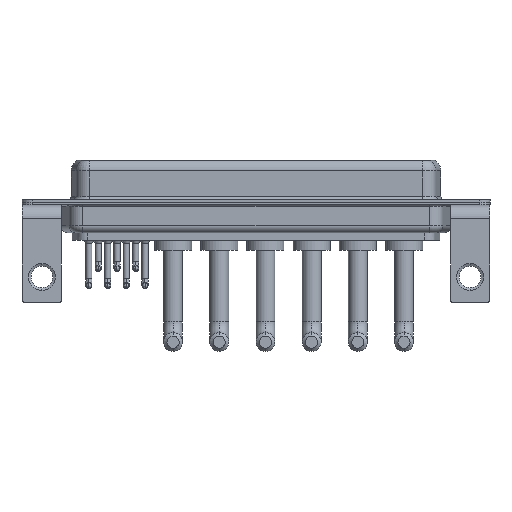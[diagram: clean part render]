
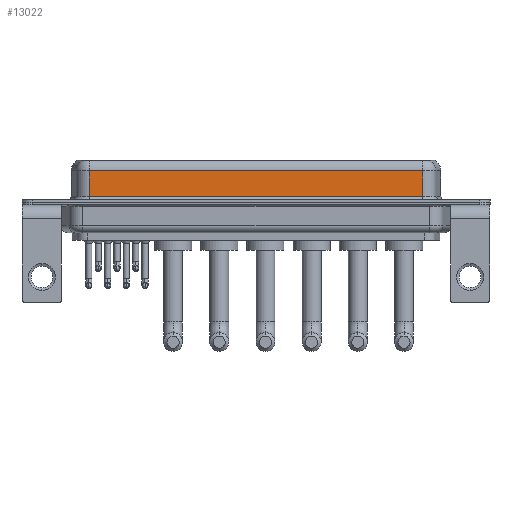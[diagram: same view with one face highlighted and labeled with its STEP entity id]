
A CAD part, front view. The second image highlights one B-rep face of the part: STEP entity #13022.
In plain terms, the highlighted planar face has unit normal (0, -1, 0).
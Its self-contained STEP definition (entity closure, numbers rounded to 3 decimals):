
#27 = CARTESIAN_POINT ( 'NONE',  ( 56.462, -3.95, 4.65 ) ) ;
#78 = AXIS2_PLACEMENT_3D ( 'NONE', #16535, #6157, #426 ) ;
#381 = ORIENTED_EDGE ( 'NONE', *, *, #7576, .T. ) ;
#426 = DIRECTION ( 'NONE',  ( 0., 0., 1. ) ) ;
#2148 = VERTEX_POINT ( 'NONE', #16836 ) ;
#2538 = EDGE_LOOP ( 'NONE', ( #10037, #14525, #13976, #381 ) ) ;
#3032 = CARTESIAN_POINT ( 'NONE',  ( 7.038, -3.95, 0.9 ) ) ;
#3276 = VERTEX_POINT ( 'NONE', #14830 ) ;
#3514 = LINE ( 'NONE', #6420, #16282 ) ;
#5369 = LINE ( 'NONE', #9836, #5472 ) ;
#5472 = VECTOR ( 'NONE', #9544, 1000. ) ;
#5866 = DIRECTION ( 'NONE',  ( -1., 0., 0. ) ) ;
#6157 = DIRECTION ( 'NONE',  ( 0., 1., 0. ) ) ;
#6420 = CARTESIAN_POINT ( 'NONE',  ( 56.462, -3.95, 0.9 ) ) ;
#7576 = EDGE_CURVE ( 'NONE', #16325, #2148, #3514, .T. ) ;
#8574 = CARTESIAN_POINT ( 'NONE',  ( 56.462, -3.95, 6.4 ) ) ;
#9326 = DIRECTION ( 'NONE',  ( 1., 0., 0. ) ) ;
#9544 = DIRECTION ( 'NONE',  ( 0., 0., -1. ) ) ;
#9836 = CARTESIAN_POINT ( 'NONE',  ( 7.038, -3.95, 6.4 ) ) ;
#10037 = ORIENTED_EDGE ( 'NONE', *, *, #13389, .F. ) ;
#10908 = FACE_OUTER_BOUND ( 'NONE', #2538, .T. ) ;
#12596 = VERTEX_POINT ( 'NONE', #13663 ) ;
#12781 = EDGE_CURVE ( 'NONE', #3276, #12596, #13325, .T. ) ;
#13022 = ADVANCED_FACE ( 'NONE', ( #10908 ), #13520, .F. ) ;
#13325 = LINE ( 'NONE', #27, #17123 ) ;
#13389 = EDGE_CURVE ( 'NONE', #3276, #2148, #15934, .T. ) ;
#13520 = PLANE ( 'NONE',  #78 ) ;
#13663 = CARTESIAN_POINT ( 'NONE',  ( 7.038, -3.95, 4.65 ) ) ;
#13976 = ORIENTED_EDGE ( 'NONE', *, *, #17702, .T. ) ;
#14525 = ORIENTED_EDGE ( 'NONE', *, *, #12781, .T. ) ;
#14830 = CARTESIAN_POINT ( 'NONE',  ( 56.462, -3.95, 4.65 ) ) ;
#15901 = VECTOR ( 'NONE', #19051, 1000. ) ;
#15934 = LINE ( 'NONE', #8574, #15901 ) ;
#16282 = VECTOR ( 'NONE', #9326, 1000. ) ;
#16325 = VERTEX_POINT ( 'NONE', #3032 ) ;
#16535 = CARTESIAN_POINT ( 'NONE',  ( 56.462, -3.95, 6.4 ) ) ;
#16836 = CARTESIAN_POINT ( 'NONE',  ( 56.462, -3.95, 0.9 ) ) ;
#17123 = VECTOR ( 'NONE', #5866, 1000. ) ;
#17702 = EDGE_CURVE ( 'NONE', #12596, #16325, #5369, .T. ) ;
#19051 = DIRECTION ( 'NONE',  ( 0., 0., -1. ) ) ;
